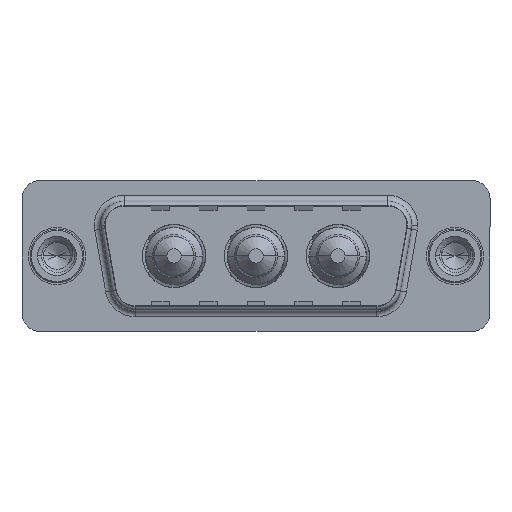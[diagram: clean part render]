
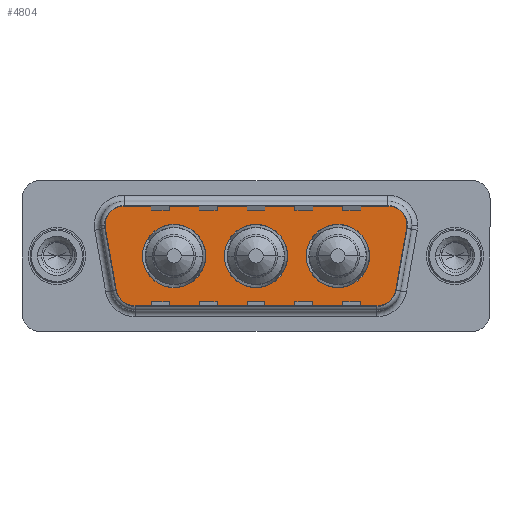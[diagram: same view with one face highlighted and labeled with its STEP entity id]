
A CAD part, top view. The second image highlights one B-rep face of the part: STEP entity #4804.
In plain terms, the highlighted planar face has unit normal (0, 0, 1).
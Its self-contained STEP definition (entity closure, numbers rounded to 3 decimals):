
#43 = DIRECTION ( 'NONE',  ( 0., 0., 1. ) ) ;
#82 = ORIENTED_EDGE ( 'NONE', *, *, #13420, .F. ) ;
#189 = ORIENTED_EDGE ( 'NONE', *, *, #10335, .T. ) ;
#272 = VECTOR ( 'NONE', #2192, 1000. ) ;
#335 = EDGE_CURVE ( 'NONE', #8692, #10020, #12983, .T. ) ;
#416 = ORIENTED_EDGE ( 'NONE', *, *, #5108, .T. ) ;
#439 = DIRECTION ( 'NONE',  ( 0.174, -0.985, 0. ) ) ;
#714 = CARTESIAN_POINT ( 'NONE',  ( 3.441, 2.553, 0. ) ) ;
#748 = AXIS2_PLACEMENT_3D ( 'NONE', #9600, #10386, #8564 ) ;
#951 = EDGE_LOOP ( 'NONE', ( #13978, #2107 ) ) ;
#995 = EDGE_CURVE ( 'NONE', #3251, #1517, #5352, .T. ) ;
#1164 = CARTESIAN_POINT ( 'NONE',  ( 16.65, 0., 0. ) ) ;
#1169 = LINE ( 'NONE', #4664, #6458 ) ;
#1306 = EDGE_LOOP ( 'NONE', ( #9838, #14030, #189, #12640, #4296, #3172, #416, #9464, #5617 ) ) ;
#1517 = VERTEX_POINT ( 'NONE', #10615 ) ;
#1567 = CARTESIAN_POINT ( 'NONE',  ( 23.5, 0., 0. ) ) ;
#1613 = LINE ( 'NONE', #714, #13066 ) ;
#1647 = CIRCLE ( 'NONE', #8431, 2. ) ;
#1785 = CIRCLE ( 'NONE', #5390, 2.65 ) ;
#1801 = CARTESIAN_POINT ( 'NONE',  ( 27.889, 2.9, 0. ) ) ;
#1841 = CARTESIAN_POINT ( 'NONE',  ( 7.15, 0., 0. ) ) ;
#1984 = VERTEX_POINT ( 'NONE', #2543 ) ;
#2107 = ORIENTED_EDGE ( 'NONE', *, *, #3512, .F. ) ;
#2192 = DIRECTION ( 'NONE',  ( -1., 0., 0. ) ) ;
#2283 = DIRECTION ( 'NONE',  ( 1., 0., 0. ) ) ;
#2316 = DIRECTION ( 'NONE',  ( 1., 0., 0. ) ) ;
#2388 = VECTOR ( 'NONE', #2316, 1000. ) ;
#2490 = FACE_BOUND ( 'NONE', #6748, .T. ) ;
#2543 = CARTESIAN_POINT ( 'NONE',  ( 26.15, 0., 0. ) ) ;
#2686 = DIRECTION ( 'NONE',  ( 1., 0., 0. ) ) ;
#2839 = DIRECTION ( 'NONE',  ( 1., 0., 0. ) ) ;
#2902 = CARTESIAN_POINT ( 'NONE',  ( 5.411, 4.9, 0. ) ) ;
#2913 = DIRECTION ( 'NONE',  ( -1., 0., 0. ) ) ;
#3141 = DIRECTION ( 'NONE',  ( 0., 0., 1. ) ) ;
#3172 = ORIENTED_EDGE ( 'NONE', *, *, #335, .T. ) ;
#3202 = ORIENTED_EDGE ( 'NONE', *, *, #14365, .F. ) ;
#3251 = VERTEX_POINT ( 'NONE', #7166 ) ;
#3512 = EDGE_CURVE ( 'NONE', #8705, #7519, #13615, .T. ) ;
#3817 = VERTEX_POINT ( 'NONE', #4011 ) ;
#3882 = DIRECTION ( 'NONE',  ( 1., 0., 0. ) ) ;
#4011 = CARTESIAN_POINT ( 'NONE',  ( 14., 0., 0. ) ) ;
#4063 = CIRCLE ( 'NONE', #7537, 2. ) ;
#4158 = DIRECTION ( 'NONE',  ( 0., 0., 1. ) ) ;
#4296 = ORIENTED_EDGE ( 'NONE', *, *, #9601, .T. ) ;
#4412 = AXIS2_PLACEMENT_3D ( 'NONE', #10007, #3141, #11143 ) ;
#4429 = DIRECTION ( 'NONE',  ( 0., 0., 1. ) ) ;
#4539 = AXIS2_PLACEMENT_3D ( 'NONE', #14446, #14720, #14768 ) ;
#4664 = CARTESIAN_POINT ( 'NONE',  ( 29.859, 2.553, 0. ) ) ;
#4804 = ADVANCED_FACE ( 'NONE', ( #2490, #8215, #11258, #5098 ), #13931, .T. ) ;
#5098 = FACE_OUTER_BOUND ( 'NONE', #1306, .T. ) ;
#5108 = EDGE_CURVE ( 'NONE', #10020, #7776, #1613, .T. ) ;
#5114 = CARTESIAN_POINT ( 'NONE',  ( 9.8, 0., 0. ) ) ;
#5340 = CARTESIAN_POINT ( 'NONE',  ( 16.65, 0., 0. ) ) ;
#5352 = LINE ( 'NONE', #6526, #2388 ) ;
#5390 = AXIS2_PLACEMENT_3D ( 'NONE', #1567, #9548, #2686 ) ;
#5531 = DIRECTION ( 'NONE',  ( 0., 0., 1. ) ) ;
#5546 = AXIS2_PLACEMENT_3D ( 'NONE', #12472, #5531, #13622 ) ;
#5589 = AXIS2_PLACEMENT_3D ( 'NONE', #1164, #9145, #2283 ) ;
#5617 = ORIENTED_EDGE ( 'NONE', *, *, #995, .T. ) ;
#5969 = CARTESIAN_POINT ( 'NONE',  ( 23.5, 0., 0. ) ) ;
#6333 = CARTESIAN_POINT ( 'NONE',  ( 9.8, 0., 0. ) ) ;
#6458 = VECTOR ( 'NONE', #13825, 1000. ) ;
#6520 = DIRECTION ( 'NONE',  ( 1., 0., 0. ) ) ;
#6526 = CARTESIAN_POINT ( 'NONE',  ( 6.434, -4.9, 0. ) ) ;
#6748 = EDGE_LOOP ( 'NONE', ( #3202, #8048 ) ) ;
#7118 = DIRECTION ( 'NONE',  ( 1., 0., 0. ) ) ;
#7166 = CARTESIAN_POINT ( 'NONE',  ( 6.434, -4.9, 0. ) ) ;
#7388 = CARTESIAN_POINT ( 'NONE',  ( 4.464, -3.247, 0. ) ) ;
#7442 = EDGE_CURVE ( 'NONE', #7519, #8705, #9757, .T. ) ;
#7489 = ORIENTED_EDGE ( 'NONE', *, *, #14135, .F. ) ;
#7519 = VERTEX_POINT ( 'NONE', #13200 ) ;
#7537 = AXIS2_PLACEMENT_3D ( 'NONE', #1801, #9785, #2913 ) ;
#7596 = VERTEX_POINT ( 'NONE', #13796 ) ;
#7776 = VERTEX_POINT ( 'NONE', #7388 ) ;
#8048 = ORIENTED_EDGE ( 'NONE', *, *, #13964, .F. ) ;
#8158 = EDGE_CURVE ( 'NONE', #12515, #10563, #1169, .T. ) ;
#8215 = FACE_BOUND ( 'NONE', #10527, .T. ) ;
#8431 = AXIS2_PLACEMENT_3D ( 'NONE', #11352, #4429, #12511 ) ;
#8564 = DIRECTION ( 'NONE',  ( 1., 0., 0. ) ) ;
#8626 = AXIS2_PLACEMENT_3D ( 'NONE', #6333, #43, #2839 ) ;
#8692 = VERTEX_POINT ( 'NONE', #2902 ) ;
#8705 = VERTEX_POINT ( 'NONE', #1841 ) ;
#8750 = VERTEX_POINT ( 'NONE', #13277 ) ;
#8816 = CIRCLE ( 'NONE', #5546, 2. ) ;
#8902 = CIRCLE ( 'NONE', #5589, 2.65 ) ;
#8934 = EDGE_CURVE ( 'NONE', #7776, #3251, #8816, .T. ) ;
#9037 = CARTESIAN_POINT ( 'NONE',  ( 28.836, -3.247, 0. ) ) ;
#9124 = CIRCLE ( 'NONE', #14536, 2.65 ) ;
#9145 = DIRECTION ( 'NONE',  ( 0., 0., 1. ) ) ;
#9154 = AXIS2_PLACEMENT_3D ( 'NONE', #5114, #4158, #3882 ) ;
#9464 = ORIENTED_EDGE ( 'NONE', *, *, #8934, .T. ) ;
#9548 = DIRECTION ( 'NONE',  ( 0., 0., 1. ) ) ;
#9600 = CARTESIAN_POINT ( 'NONE',  ( 5.411, 2.9, 0. ) ) ;
#9601 = EDGE_CURVE ( 'NONE', #8750, #8692, #9732, .T. ) ;
#9732 = LINE ( 'NONE', #11342, #272 ) ;
#9757 = CIRCLE ( 'NONE', #9154, 2.65 ) ;
#9785 = DIRECTION ( 'NONE',  ( 0., 0., 1. ) ) ;
#9838 = ORIENTED_EDGE ( 'NONE', *, *, #11821, .T. ) ;
#10007 = CARTESIAN_POINT ( 'NONE',  ( 27.889, 2.9, 0. ) ) ;
#10020 = VERTEX_POINT ( 'NONE', #11901 ) ;
#10335 = EDGE_CURVE ( 'NONE', #10563, #10800, #12072, .T. ) ;
#10386 = DIRECTION ( 'NONE',  ( 0., 0., 1. ) ) ;
#10527 = EDGE_LOOP ( 'NONE', ( #7489, #82 ) ) ;
#10563 = VERTEX_POINT ( 'NONE', #11627 ) ;
#10615 = CARTESIAN_POINT ( 'NONE',  ( 26.866, -4.9, 0. ) ) ;
#10800 = VERTEX_POINT ( 'NONE', #14226 ) ;
#11044 = VERTEX_POINT ( 'NONE', #14550 ) ;
#11143 = DIRECTION ( 'NONE',  ( -1., 0., 0. ) ) ;
#11258 = FACE_BOUND ( 'NONE', #951, .T. ) ;
#11342 = CARTESIAN_POINT ( 'NONE',  ( 5.411, 4.9, 0. ) ) ;
#11352 = CARTESIAN_POINT ( 'NONE',  ( 26.866, -2.9, 0. ) ) ;
#11627 = CARTESIAN_POINT ( 'NONE',  ( 29.859, 2.553, 0. ) ) ;
#11821 = EDGE_CURVE ( 'NONE', #1517, #12515, #1647, .T. ) ;
#11901 = CARTESIAN_POINT ( 'NONE',  ( 3.441, 2.553, 0. ) ) ;
#12072 = CIRCLE ( 'NONE', #4412, 2. ) ;
#12472 = CARTESIAN_POINT ( 'NONE',  ( 6.434, -2.9, 0. ) ) ;
#12511 = DIRECTION ( 'NONE',  ( 1., 0., 0. ) ) ;
#12515 = VERTEX_POINT ( 'NONE', #9037 ) ;
#12573 = AXIS2_PLACEMENT_3D ( 'NONE', #5969, #14027, #7118 ) ;
#12640 = ORIENTED_EDGE ( 'NONE', *, *, #12841, .T. ) ;
#12841 = EDGE_CURVE ( 'NONE', #10800, #8750, #4063, .T. ) ;
#12983 = CIRCLE ( 'NONE', #748, 2. ) ;
#13066 = VECTOR ( 'NONE', #439, 1000. ) ;
#13200 = CARTESIAN_POINT ( 'NONE',  ( 12.45, 0., 0. ) ) ;
#13218 = CIRCLE ( 'NONE', #12573, 2.65 ) ;
#13277 = CARTESIAN_POINT ( 'NONE',  ( 27.889, 4.9, 0. ) ) ;
#13420 = EDGE_CURVE ( 'NONE', #11044, #1984, #1785, .T. ) ;
#13421 = DIRECTION ( 'NONE',  ( 0., 0., 1. ) ) ;
#13615 = CIRCLE ( 'NONE', #8626, 2.65 ) ;
#13622 = DIRECTION ( 'NONE',  ( -1., 0., 0. ) ) ;
#13796 = CARTESIAN_POINT ( 'NONE',  ( 19.3, 0., 0. ) ) ;
#13825 = DIRECTION ( 'NONE',  ( 0.174, 0.985, 0. ) ) ;
#13931 = PLANE ( 'NONE',  #4539 ) ;
#13964 = EDGE_CURVE ( 'NONE', #3817, #7596, #8902, .T. ) ;
#13978 = ORIENTED_EDGE ( 'NONE', *, *, #7442, .F. ) ;
#14027 = DIRECTION ( 'NONE',  ( 0., 0., 1. ) ) ;
#14030 = ORIENTED_EDGE ( 'NONE', *, *, #8158, .T. ) ;
#14135 = EDGE_CURVE ( 'NONE', #1984, #11044, #13218, .T. ) ;
#14226 = CARTESIAN_POINT ( 'NONE',  ( 29.889, 2.9, 0. ) ) ;
#14365 = EDGE_CURVE ( 'NONE', #7596, #3817, #9124, .T. ) ;
#14446 = CARTESIAN_POINT ( 'NONE',  ( 26.866, -2.9, 0. ) ) ;
#14536 = AXIS2_PLACEMENT_3D ( 'NONE', #5340, #13421, #6520 ) ;
#14550 = CARTESIAN_POINT ( 'NONE',  ( 20.85, 0., 0. ) ) ;
#14720 = DIRECTION ( 'NONE',  ( 0., 0., 1. ) ) ;
#14768 = DIRECTION ( 'NONE',  ( 1., 0., 0. ) ) ;
